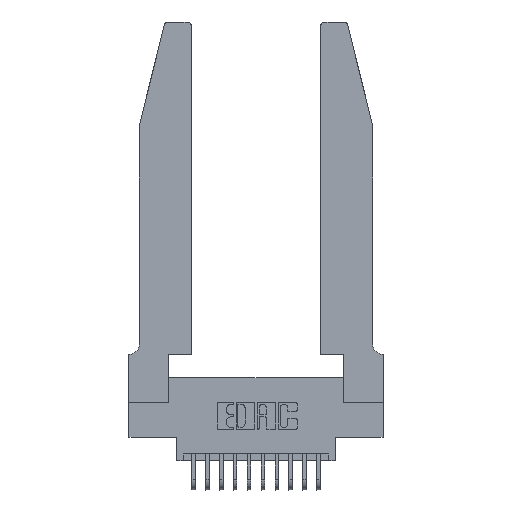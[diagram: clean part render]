
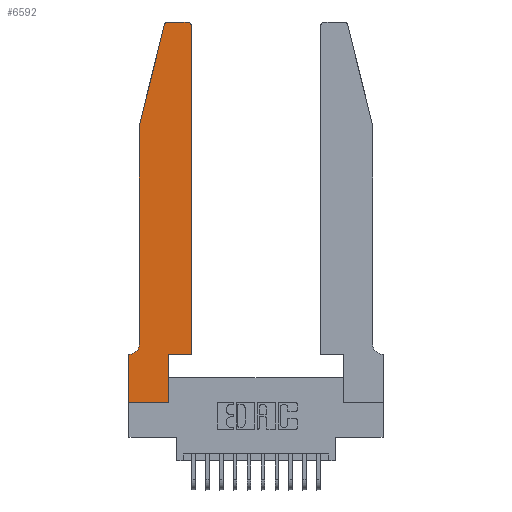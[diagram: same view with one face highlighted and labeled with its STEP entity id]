
A CAD part, top view. The second image highlights one B-rep face of the part: STEP entity #6592.
In plain terms, the highlighted planar face has unit normal (0, 0, 1).
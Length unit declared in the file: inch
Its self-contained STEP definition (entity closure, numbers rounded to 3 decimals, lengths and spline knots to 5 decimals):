
#582 = CARTESIAN_POINT ( 'NONE',  ( 0.0755, 0.35, 0.37 ) ) ;
#596 = DIRECTION ( 'NONE',  ( 0., 0., 1. ) ) ;
#853 = VERTEX_POINT ( 'NONE', #2811 ) ;
#929 = EDGE_CURVE ( 'NONE', #853, #8086, #9715, .T. ) ;
#1045 = CARTESIAN_POINT ( 'NONE',  ( 0.2605, 2.75, 0.37 ) ) ;
#1432 = EDGE_CURVE ( 'NONE', #5598, #853, #2839, .T. ) ;
#1446 = AXIS2_PLACEMENT_3D ( 'NONE', #6079, #6064, #6058 ) ;
#1462 = EDGE_LOOP ( 'NONE', ( #7698, #3144, #7994, #5200, #15581, #12941, #1662, #5804, #3687, #13291, #10098, #9072 ) ) ;
#1492 = VERTEX_POINT ( 'NONE', #16567 ) ;
#1662 = ORIENTED_EDGE ( 'NONE', *, *, #13747, .T. ) ;
#1759 = DIRECTION ( 'NONE',  ( 0., 1., 0. ) ) ;
#2445 = CARTESIAN_POINT ( 'NONE',  ( 0.0055, 0.42, 0.37 ) ) ;
#2697 = VECTOR ( 'NONE', #13076, 39.37008 ) ;
#2811 = CARTESIAN_POINT ( 'NONE',  ( 0.25487, 2.72718, 0.37 ) ) ;
#2839 = CIRCLE ( 'NONE', #1446, 0.03 ) ;
#2957 = CARTESIAN_POINT ( 'NONE',  ( 0., 0., 0.37 ) ) ;
#3014 = CARTESIAN_POINT ( 'NONE',  ( 0., 0., 0.37 ) ) ;
#3144 = ORIENTED_EDGE ( 'NONE', *, *, #1432, .T. ) ;
#3687 = ORIENTED_EDGE ( 'NONE', *, *, #12783, .T. ) ;
#3695 = DIRECTION ( 'NONE',  ( 1., 0., 0. ) ) ;
#3772 = LINE ( 'NONE', #1045, #13914 ) ;
#3884 = DIRECTION ( 'NONE',  ( -1., 0., 0. ) ) ;
#3961 = CARTESIAN_POINT ( 'NONE',  ( 0.0055, 0.35, 0.37 ) ) ;
#4603 = EDGE_CURVE ( 'NONE', #1492, #14099, #4793, .T. ) ;
#4793 = LINE ( 'NONE', #7390, #8280 ) ;
#4890 = CARTESIAN_POINT ( 'NONE',  ( 0.0755, 2., 0.37 ) ) ;
#5097 = VERTEX_POINT ( 'NONE', #6503 ) ;
#5167 = EDGE_CURVE ( 'NONE', #8134, #12488, #15319, .T. ) ;
#5200 = ORIENTED_EDGE ( 'NONE', *, *, #7603, .T. ) ;
#5259 = FACE_OUTER_BOUND ( 'NONE', #1462, .T. ) ;
#5260 = CARTESIAN_POINT ( 'NONE',  ( 0.0755, 0.42, 0.37 ) ) ;
#5421 = DIRECTION ( 'NONE',  ( 0., 1., 0. ) ) ;
#5444 = DIRECTION ( 'NONE',  ( 0., 0., 1. ) ) ;
#5598 = VERTEX_POINT ( 'NONE', #10501 ) ;
#5804 = ORIENTED_EDGE ( 'NONE', *, *, #5167, .T. ) ;
#5841 = VECTOR ( 'NONE', #13900, 39.37008 ) ;
#6058 = DIRECTION ( 'NONE',  ( 1., 0., 0. ) ) ;
#6064 = DIRECTION ( 'NONE',  ( 0., 0., 1. ) ) ;
#6079 = CARTESIAN_POINT ( 'NONE',  ( 0.284, 2.72, 0.37 ) ) ;
#6503 = CARTESIAN_POINT ( 'NONE',  ( 0.4205, 2.75, 0.37 ) ) ;
#6571 = DIRECTION ( 'NONE',  ( -1., 0., 0. ) ) ;
#6592 = ADVANCED_FACE ( 'NONE', ( #5259 ), #12649, .T. ) ;
#6822 = CARTESIAN_POINT ( 'NONE',  ( 0., 0.35, 0.37 ) ) ;
#6887 = VECTOR ( 'NONE', #5421, 39.37008 ) ;
#7002 = VECTOR ( 'NONE', #6571, 39.37008 ) ;
#7241 = EDGE_CURVE ( 'NONE', #14099, #12714, #18210, .T. ) ;
#7390 = CARTESIAN_POINT ( 'NONE',  ( 0.4505, 0.35, 0.37 ) ) ;
#7470 = CARTESIAN_POINT ( 'NONE',  ( 0.4505, 2.72, 0.37 ) ) ;
#7548 = LINE ( 'NONE', #2957, #2697 ) ;
#7603 = EDGE_CURVE ( 'NONE', #8086, #13506, #16658, .T. ) ;
#7656 = CARTESIAN_POINT ( 'NONE',  ( 0.2865, 0.35, 0.37 ) ) ;
#7669 = AXIS2_PLACEMENT_3D ( 'NONE', #9451, #596, #10858 ) ;
#7698 = ORIENTED_EDGE ( 'NONE', *, *, #9731, .T. ) ;
#7932 = VERTEX_POINT ( 'NONE', #3961 ) ;
#7994 = ORIENTED_EDGE ( 'NONE', *, *, #929, .T. ) ;
#8086 = VERTEX_POINT ( 'NONE', #17215 ) ;
#8134 = VERTEX_POINT ( 'NONE', #3014 ) ;
#8234 = CIRCLE ( 'NONE', #7669, 0.03 ) ;
#8280 = VECTOR ( 'NONE', #15927, 39.37008 ) ;
#8508 = VERTEX_POINT ( 'NONE', #6822 ) ;
#8527 = EDGE_CURVE ( 'NONE', #13506, #7932, #17058, .T. ) ;
#8724 = VECTOR ( 'NONE', #13519, 39.37008 ) ;
#9072 = ORIENTED_EDGE ( 'NONE', *, *, #13390, .T. ) ;
#9451 = CARTESIAN_POINT ( 'NONE',  ( 0.4205, 2.72, 0.37 ) ) ;
#9715 = LINE ( 'NONE', #16952, #5841 ) ;
#9731 = EDGE_CURVE ( 'NONE', #5097, #5598, #3772, .T. ) ;
#9769 = CARTESIAN_POINT ( 'NONE',  ( 0.4505, 0.35, 0.37 ) ) ;
#10098 = ORIENTED_EDGE ( 'NONE', *, *, #7241, .T. ) ;
#10501 = CARTESIAN_POINT ( 'NONE',  ( 0.284, 2.75, 0.37 ) ) ;
#10858 = DIRECTION ( 'NONE',  ( 1., 0., 0. ) ) ;
#12456 = CARTESIAN_POINT ( 'NONE',  ( 0.4505, 0.35, 0.37 ) ) ;
#12488 = VERTEX_POINT ( 'NONE', #12645 ) ;
#12578 = DIRECTION ( 'NONE',  ( 0., 0., -1. ) ) ;
#12645 = CARTESIAN_POINT ( 'NONE',  ( 0.2865, 0., 0.37 ) ) ;
#12649 = PLANE ( 'NONE',  #17325 ) ;
#12714 = VERTEX_POINT ( 'NONE', #7470 ) ;
#12783 = EDGE_CURVE ( 'NONE', #12488, #1492, #18176, .T. ) ;
#12941 = ORIENTED_EDGE ( 'NONE', *, *, #15614, .T. ) ;
#13076 = DIRECTION ( 'NONE',  ( 0., -1., 0. ) ) ;
#13291 = ORIENTED_EDGE ( 'NONE', *, *, #4603, .T. ) ;
#13390 = EDGE_CURVE ( 'NONE', #12714, #5097, #8234, .T. ) ;
#13506 = VERTEX_POINT ( 'NONE', #5260 ) ;
#13519 = DIRECTION ( 'NONE',  ( 0., -1., 0. ) ) ;
#13747 = EDGE_CURVE ( 'NONE', #8508, #8134, #7548, .T. ) ;
#13900 = DIRECTION ( 'NONE',  ( -0.239, -0.971, 0. ) ) ;
#13914 = VECTOR ( 'NONE', #16963, 39.37008 ) ;
#13960 = VECTOR ( 'NONE', #1759, 39.37008 ) ;
#14033 = CARTESIAN_POINT ( 'NONE',  ( 0., 0.35, 0.37 ) ) ;
#14099 = VERTEX_POINT ( 'NONE', #12456 ) ;
#14428 = VECTOR ( 'NONE', #3695, 39.37008 ) ;
#14555 = LINE ( 'NONE', #582, #7002 ) ;
#15319 = LINE ( 'NONE', #16574, #14428 ) ;
#15454 = DIRECTION ( 'NONE',  ( 1., 0., 0. ) ) ;
#15581 = ORIENTED_EDGE ( 'NONE', *, *, #8527, .T. ) ;
#15614 = EDGE_CURVE ( 'NONE', #7932, #8508, #14555, .T. ) ;
#15927 = DIRECTION ( 'NONE',  ( 1., 0., 0. ) ) ;
#16507 = AXIS2_PLACEMENT_3D ( 'NONE', #2445, #12578, #3884 ) ;
#16567 = CARTESIAN_POINT ( 'NONE',  ( 0.2865, 0.35, 0.37 ) ) ;
#16574 = CARTESIAN_POINT ( 'NONE',  ( 0., 0., 0.37 ) ) ;
#16658 = LINE ( 'NONE', #4890, #8724 ) ;
#16952 = CARTESIAN_POINT ( 'NONE',  ( 0.0755, 2., 0.37 ) ) ;
#16963 = DIRECTION ( 'NONE',  ( -1., 0., 0. ) ) ;
#17058 = CIRCLE ( 'NONE', #16507, 0.07 ) ;
#17215 = CARTESIAN_POINT ( 'NONE',  ( 0.0755, 2., 0.37 ) ) ;
#17325 = AXIS2_PLACEMENT_3D ( 'NONE', #14033, #5444, #15454 ) ;
#18176 = LINE ( 'NONE', #7656, #13960 ) ;
#18210 = LINE ( 'NONE', #9769, #6887 ) ;
